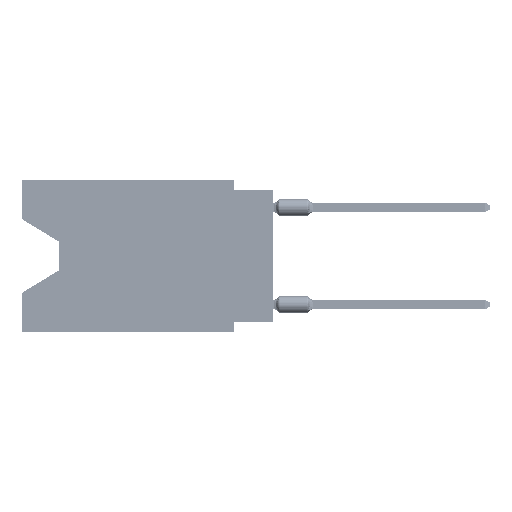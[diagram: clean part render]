
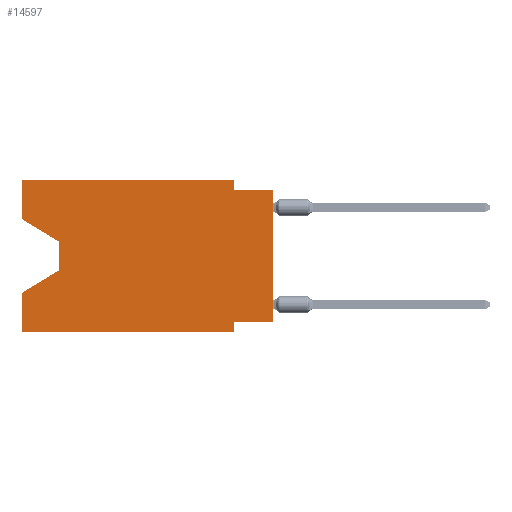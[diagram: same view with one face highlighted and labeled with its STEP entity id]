
A CAD part, left-side view. The second image highlights one B-rep face of the part: STEP entity #14597.
In plain terms, the highlighted planar face has unit normal (-1, 0, 0).
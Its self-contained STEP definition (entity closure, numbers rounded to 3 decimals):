
#250 = CARTESIAN_POINT ( 'NONE',  ( 0., 16.383, -9.906 ) ) ;
#510 = CARTESIAN_POINT ( 'NONE',  ( 0., 16.383, 0. ) ) ;
#1024 = DIRECTION ( 'NONE',  ( 0., 0., 1. ) ) ;
#1414 = ORIENTED_EDGE ( 'NONE', *, *, #43323, .F. ) ;
#1816 = VECTOR ( 'NONE', #18745, 1000. ) ;
#2867 = LINE ( 'NONE', #74958, #32858 ) ;
#3211 = CARTESIAN_POINT ( 'NONE',  ( 0., 13.97, -5.893 ) ) ;
#4485 = CARTESIAN_POINT ( 'NONE',  ( 0., 16.383, -2.546 ) ) ;
#5436 = EDGE_CURVE ( 'NONE', #18263, #9376, #10835, .T. ) ;
#6408 = FACE_OUTER_BOUND ( 'NONE', #31966, .T. ) ;
#7144 = EDGE_CURVE ( 'NONE', #10950, #29599, #18651, .T. ) ;
#8145 = ORIENTED_EDGE ( 'NONE', *, *, #49540, .T. ) ;
#8456 = EDGE_CURVE ( 'NONE', #10950, #23218, #12768, .T. ) ;
#8459 = ORIENTED_EDGE ( 'NONE', *, *, #66793, .T. ) ;
#8520 = DIRECTION ( 'NONE',  ( 0., -0.855, -0.519 ) ) ;
#9376 = VERTEX_POINT ( 'NONE', #62689 ) ;
#9586 = VECTOR ( 'NONE', #9715, 1000. ) ;
#9715 = DIRECTION ( 'NONE',  ( 0., 0., 1. ) ) ;
#10835 = LINE ( 'NONE', #59826, #47207 ) ;
#10950 = VERTEX_POINT ( 'NONE', #34822 ) ;
#10954 = CARTESIAN_POINT ( 'NONE',  ( 0., 2.54, -9.906 ) ) ;
#12768 = LINE ( 'NONE', #60579, #67868 ) ;
#13241 = CARTESIAN_POINT ( 'NONE',  ( 0., 0., -9.271 ) ) ;
#14597 = ADVANCED_FACE ( 'NONE', ( #6408 ), #54202, .F. ) ;
#15040 = CARTESIAN_POINT ( 'NONE',  ( 0., 0., -0.635 ) ) ;
#16156 = DIRECTION ( 'NONE',  ( 0., 0.855, -0.519 ) ) ;
#17638 = DIRECTION ( 'NONE',  ( 0., 0., -1. ) ) ;
#18263 = VERTEX_POINT ( 'NONE', #52742 ) ;
#18651 = LINE ( 'NONE', #250, #48775 ) ;
#18745 = DIRECTION ( 'NONE',  ( 0., 1., 0. ) ) ;
#20699 = VECTOR ( 'NONE', #8520, 1000. ) ;
#22750 = VERTEX_POINT ( 'NONE', #44359 ) ;
#23205 = DIRECTION ( 'NONE',  ( 0., 0., -1. ) ) ;
#23218 = VERTEX_POINT ( 'NONE', #55274 ) ;
#27359 = LINE ( 'NONE', #32853, #9586 ) ;
#27721 = CARTESIAN_POINT ( 'NONE',  ( 0., 16.383, 0. ) ) ;
#29076 = CARTESIAN_POINT ( 'NONE',  ( 0., 2.54, 0. ) ) ;
#29081 = ORIENTED_EDGE ( 'NONE', *, *, #54662, .F. ) ;
#29599 = VERTEX_POINT ( 'NONE', #40382 ) ;
#30110 = LINE ( 'NONE', #13241, #1816 ) ;
#30170 = LINE ( 'NONE', #10954, #67071 ) ;
#31746 = VECTOR ( 'NONE', #54583, 1000. ) ;
#31966 = EDGE_LOOP ( 'NONE', ( #8459, #31994, #8145, #32543, #77394, #70063, #46277, #45835, #52197, #1414, #29081, #69182 ) ) ;
#31994 = ORIENTED_EDGE ( 'NONE', *, *, #73849, .T. ) ;
#32543 = ORIENTED_EDGE ( 'NONE', *, *, #8456, .F. ) ;
#32853 = CARTESIAN_POINT ( 'NONE',  ( 0., 0., 0. ) ) ;
#32858 = VECTOR ( 'NONE', #16156, 1000. ) ;
#34822 = CARTESIAN_POINT ( 'NONE',  ( 0., 16.383, -9.906 ) ) ;
#35840 = VERTEX_POINT ( 'NONE', #73787 ) ;
#36534 = CARTESIAN_POINT ( 'NONE',  ( 0., 13.97, -4.013 ) ) ;
#36548 = EDGE_CURVE ( 'NONE', #22750, #59931, #30110, .T. ) ;
#37082 = VERTEX_POINT ( 'NONE', #3211 ) ;
#39641 = VECTOR ( 'NONE', #77122, 1000. ) ;
#40382 = CARTESIAN_POINT ( 'NONE',  ( 0., 2.54, -9.906 ) ) ;
#41667 = DIRECTION ( 'NONE',  ( 1., 0., 0. ) ) ;
#42037 = LINE ( 'NONE', #29076, #51309 ) ;
#43323 = EDGE_CURVE ( 'NONE', #35840, #67305, #42037, .T. ) ;
#44359 = CARTESIAN_POINT ( 'NONE',  ( 0., 0., -9.271 ) ) ;
#45749 = DIRECTION ( 'NONE',  ( 0., -1., 0. ) ) ;
#45835 = ORIENTED_EDGE ( 'NONE', *, *, #70759, .T. ) ;
#46277 = ORIENTED_EDGE ( 'NONE', *, *, #36548, .F. ) ;
#47207 = VECTOR ( 'NONE', #66095, 1000. ) ;
#48053 = DIRECTION ( 'NONE',  ( 0., -1., 0. ) ) ;
#48319 = DIRECTION ( 'NONE',  ( 0., 0., -1. ) ) ;
#48775 = VECTOR ( 'NONE', #48053, 1000. ) ;
#49540 = EDGE_CURVE ( 'NONE', #37082, #23218, #2867, .T. ) ;
#51309 = VECTOR ( 'NONE', #23205, 1000. ) ;
#51979 = VERTEX_POINT ( 'NONE', #15040 ) ;
#52022 = LINE ( 'NONE', #27721, #57392 ) ;
#52197 = ORIENTED_EDGE ( 'NONE', *, *, #70855, .F. ) ;
#52615 = EDGE_CURVE ( 'NONE', #59931, #29599, #30170, .T. ) ;
#52742 = CARTESIAN_POINT ( 'NONE',  ( 0., 16.383, -2.546 ) ) ;
#53216 = CARTESIAN_POINT ( 'NONE',  ( 0., 0., -0.635 ) ) ;
#53913 = CARTESIAN_POINT ( 'NONE',  ( 0., 13.97, -4.013 ) ) ;
#54202 = PLANE ( 'NONE',  #60796 ) ;
#54583 = DIRECTION ( 'NONE',  ( 0., 0., -1. ) ) ;
#54662 = EDGE_CURVE ( 'NONE', #9376, #35840, #52022, .T. ) ;
#55274 = CARTESIAN_POINT ( 'NONE',  ( 0., 16.383, -7.36 ) ) ;
#56359 = VERTEX_POINT ( 'NONE', #53913 ) ;
#57392 = VECTOR ( 'NONE', #45749, 1000. ) ;
#57775 = LINE ( 'NONE', #4485, #20699 ) ;
#59826 = CARTESIAN_POINT ( 'NONE',  ( 0., 16.383, 0. ) ) ;
#59931 = VERTEX_POINT ( 'NONE', #76802 ) ;
#60579 = CARTESIAN_POINT ( 'NONE',  ( 0., 16.383, 0. ) ) ;
#60796 = AXIS2_PLACEMENT_3D ( 'NONE', #510, #41667, #48319 ) ;
#62689 = CARTESIAN_POINT ( 'NONE',  ( 0., 16.383, 0. ) ) ;
#66095 = DIRECTION ( 'NONE',  ( 0., 0., 1. ) ) ;
#66793 = EDGE_CURVE ( 'NONE', #18263, #56359, #57775, .T. ) ;
#67071 = VECTOR ( 'NONE', #17638, 1000. ) ;
#67305 = VERTEX_POINT ( 'NONE', #77266 ) ;
#67868 = VECTOR ( 'NONE', #1024, 1000. ) ;
#69182 = ORIENTED_EDGE ( 'NONE', *, *, #5436, .F. ) ;
#70063 = ORIENTED_EDGE ( 'NONE', *, *, #52615, .F. ) ;
#70759 = EDGE_CURVE ( 'NONE', #22750, #51979, #27359, .T. ) ;
#70855 = EDGE_CURVE ( 'NONE', #67305, #51979, #71654, .T. ) ;
#71654 = LINE ( 'NONE', #53216, #39641 ) ;
#72220 = LINE ( 'NONE', #36534, #31746 ) ;
#73787 = CARTESIAN_POINT ( 'NONE',  ( 0., 2.54, 0. ) ) ;
#73849 = EDGE_CURVE ( 'NONE', #56359, #37082, #72220, .T. ) ;
#74958 = CARTESIAN_POINT ( 'NONE',  ( 0., 13.97, -5.893 ) ) ;
#76802 = CARTESIAN_POINT ( 'NONE',  ( 0., 2.54, -9.271 ) ) ;
#77122 = DIRECTION ( 'NONE',  ( 0., -1., 0. ) ) ;
#77266 = CARTESIAN_POINT ( 'NONE',  ( 0., 2.54, -0.635 ) ) ;
#77394 = ORIENTED_EDGE ( 'NONE', *, *, #7144, .T. ) ;
